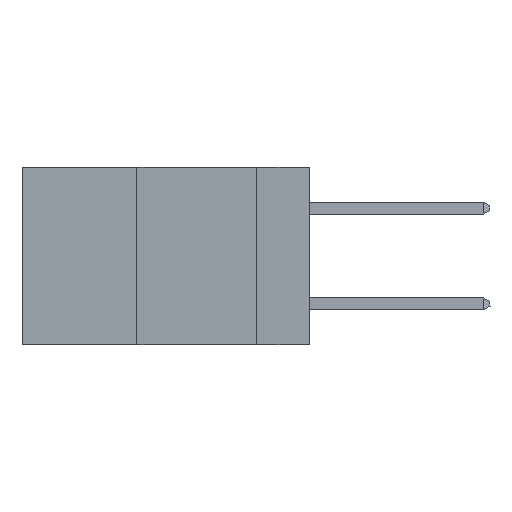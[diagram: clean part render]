
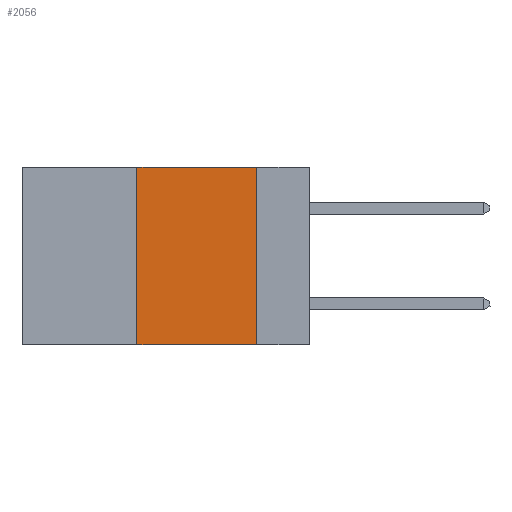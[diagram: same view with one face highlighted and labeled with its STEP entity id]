
A CAD part, left-side view. The second image highlights one B-rep face of the part: STEP entity #2056.
In plain terms, the highlighted planar face has unit normal (-1, 0, 0).
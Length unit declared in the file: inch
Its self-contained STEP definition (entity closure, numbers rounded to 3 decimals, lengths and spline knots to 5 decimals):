
#1023 = DIRECTION ( 'NONE',  ( 0., 0., -1. ) ) ;
#1083 = DIRECTION ( 'NONE',  ( 0., 0., 1. ) ) ;
#1723 = VERTEX_POINT ( 'NONE', #16414 ) ;
#2056 = ADVANCED_FACE ( 'NONE', ( #12241 ), #9941, .F. ) ;
#2169 = VERTEX_POINT ( 'NONE', #13899 ) ;
#3484 = AXIS2_PLACEMENT_3D ( 'NONE', #13264, #6421, #1023 ) ;
#6421 = DIRECTION ( 'NONE',  ( 1., 0., 0. ) ) ;
#7732 = ORIENTED_EDGE ( 'NONE', *, *, #9291, .F. ) ;
#9291 = EDGE_CURVE ( 'NONE', #1723, #23286, #16551, .T. ) ;
#9401 = EDGE_CURVE ( 'NONE', #2169, #1723, #15364, .T. ) ;
#9574 = VECTOR ( 'NONE', #14000, 39.37008 ) ;
#9702 = CARTESIAN_POINT ( 'NONE',  ( 0., 0.6, 0. ) ) ;
#9926 = EDGE_CURVE ( 'NONE', #11606, #23286, #13920, .T. ) ;
#9941 = PLANE ( 'NONE',  #3484 ) ;
#10423 = ORIENTED_EDGE ( 'NONE', *, *, #9926, .T. ) ;
#11239 = CARTESIAN_POINT ( 'NONE',  ( 0., 0.11, 0. ) ) ;
#11396 = DIRECTION ( 'NONE',  ( 0., 0., -1. ) ) ;
#11606 = VERTEX_POINT ( 'NONE', #11701 ) ;
#11644 = VECTOR ( 'NONE', #11396, 39.37008 ) ;
#11701 = CARTESIAN_POINT ( 'NONE',  ( 0., 0.36, -0.37 ) ) ;
#12241 = FACE_OUTER_BOUND ( 'NONE', #12903, .T. ) ;
#12903 = EDGE_LOOP ( 'NONE', ( #7732, #18347, #23326, #10423 ) ) ;
#13264 = CARTESIAN_POINT ( 'NONE',  ( 0., 0.6, 0. ) ) ;
#13899 = CARTESIAN_POINT ( 'NONE',  ( 0., 0.36, 0. ) ) ;
#13920 = LINE ( 'NONE', #21553, #9574 ) ;
#14000 = DIRECTION ( 'NONE',  ( 0., -1., 0. ) ) ;
#14515 = VECTOR ( 'NONE', #15415, 39.37008 ) ;
#14904 = LINE ( 'NONE', #19795, #21314 ) ;
#15364 = LINE ( 'NONE', #9702, #14515 ) ;
#15415 = DIRECTION ( 'NONE',  ( 0., -1., 0. ) ) ;
#16369 = CARTESIAN_POINT ( 'NONE',  ( 0., 0.11, -0.37 ) ) ;
#16414 = CARTESIAN_POINT ( 'NONE',  ( 0., 0.11, 0. ) ) ;
#16551 = LINE ( 'NONE', #11239, #11644 ) ;
#18347 = ORIENTED_EDGE ( 'NONE', *, *, #9401, .F. ) ;
#19498 = EDGE_CURVE ( 'NONE', #11606, #2169, #14904, .T. ) ;
#19795 = CARTESIAN_POINT ( 'NONE',  ( 0., 0.36, 0. ) ) ;
#21314 = VECTOR ( 'NONE', #1083, 39.37008 ) ;
#21553 = CARTESIAN_POINT ( 'NONE',  ( 0., 0.6, -0.37 ) ) ;
#23286 = VERTEX_POINT ( 'NONE', #16369 ) ;
#23326 = ORIENTED_EDGE ( 'NONE', *, *, #19498, .F. ) ;
